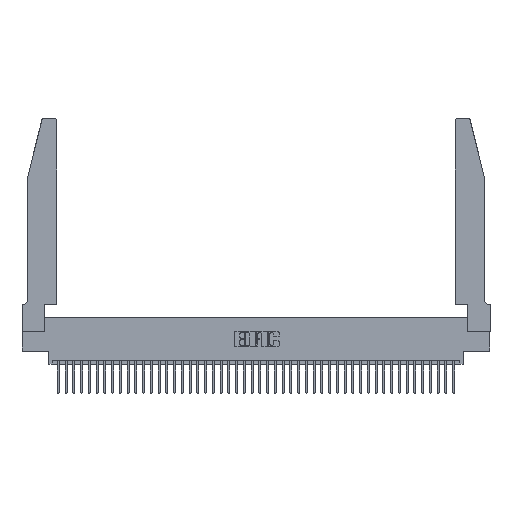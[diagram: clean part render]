
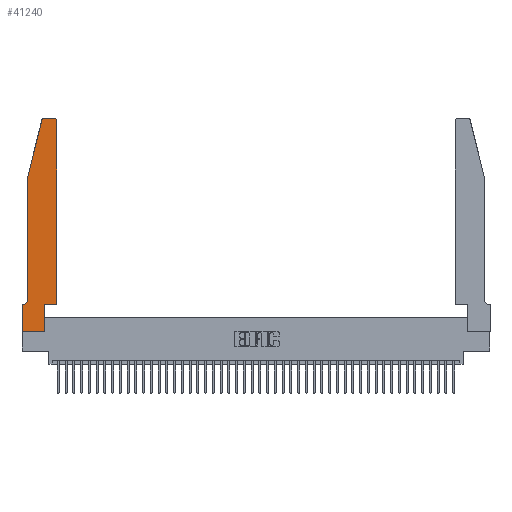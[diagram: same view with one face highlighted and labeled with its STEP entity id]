
A CAD part, top view. The second image highlights one B-rep face of the part: STEP entity #41240.
In plain terms, the highlighted planar face has unit normal (0, 0, 1).
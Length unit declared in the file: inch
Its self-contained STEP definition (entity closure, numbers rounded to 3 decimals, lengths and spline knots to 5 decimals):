
#177 = DIRECTION ( 'NONE',  ( 0., 1., 0. ) ) ;
#763 = DIRECTION ( 'NONE',  ( -0.239, -0.971, 0. ) ) ;
#1965 = CIRCLE ( 'NONE', #7921, 0.07 ) ;
#2280 = VERTEX_POINT ( 'NONE', #5767 ) ;
#2513 = ORIENTED_EDGE ( 'NONE', *, *, #29486, .T. ) ;
#2930 = DIRECTION ( 'NONE',  ( 1., 0., 0. ) ) ;
#3044 = FACE_OUTER_BOUND ( 'NONE', #36566, .T. ) ;
#3573 = AXIS2_PLACEMENT_3D ( 'NONE', #9579, #36799, #13159 ) ;
#3617 = VECTOR ( 'NONE', #177, 39.37008 ) ;
#3739 = EDGE_CURVE ( 'NONE', #2280, #36924, #19705, .T. ) ;
#4438 = CARTESIAN_POINT ( 'NONE',  ( 0.2605, 2.75, 0.37 ) ) ;
#4648 = ORIENTED_EDGE ( 'NONE', *, *, #14886, .T. ) ;
#5767 = CARTESIAN_POINT ( 'NONE',  ( 0.284, 2.75, 0.37 ) ) ;
#5982 = EDGE_CURVE ( 'NONE', #24374, #2280, #41078, .T. ) ;
#6125 = ORIENTED_EDGE ( 'NONE', *, *, #11329, .T. ) ;
#6128 = ORIENTED_EDGE ( 'NONE', *, *, #5982, .T. ) ;
#7256 = CARTESIAN_POINT ( 'NONE',  ( 0.4205, 2.72, 0.37 ) ) ;
#7770 = CARTESIAN_POINT ( 'NONE',  ( 0., 0., 0.37 ) ) ;
#7921 = AXIS2_PLACEMENT_3D ( 'NONE', #29848, #9232, #20041 ) ;
#8768 = ORIENTED_EDGE ( 'NONE', *, *, #29481, .T. ) ;
#9021 = CARTESIAN_POINT ( 'NONE',  ( 0.0055, 0.35, 0.37 ) ) ;
#9183 = VECTOR ( 'NONE', #14532, 39.37008 ) ;
#9232 = DIRECTION ( 'NONE',  ( 0., 0., -1. ) ) ;
#9338 = VECTOR ( 'NONE', #35047, 39.37008 ) ;
#9579 = CARTESIAN_POINT ( 'NONE',  ( 0., 0.35, 0.37 ) ) ;
#9632 = CARTESIAN_POINT ( 'NONE',  ( 0.284, 2.72, 0.37 ) ) ;
#9976 = VECTOR ( 'NONE', #16773, 39.37008 ) ;
#10547 = LINE ( 'NONE', #24568, #3617 ) ;
#10898 = CARTESIAN_POINT ( 'NONE',  ( 0.4505, 0.35, 0.37 ) ) ;
#11329 = EDGE_CURVE ( 'NONE', #16877, #13944, #31645, .T. ) ;
#12006 = DIRECTION ( 'NONE',  ( 1., 0., 0. ) ) ;
#12600 = ORIENTED_EDGE ( 'NONE', *, *, #39792, .T. ) ;
#13052 = CARTESIAN_POINT ( 'NONE',  ( 0.4505, 2.72, 0.37 ) ) ;
#13159 = DIRECTION ( 'NONE',  ( 1., 0., 0. ) ) ;
#13393 = EDGE_CURVE ( 'NONE', #20258, #36377, #28269, .T. ) ;
#13695 = EDGE_CURVE ( 'NONE', #18175, #24374, #19081, .T. ) ;
#13944 = VERTEX_POINT ( 'NONE', #23551 ) ;
#14532 = DIRECTION ( 'NONE',  ( 1., 0., 0. ) ) ;
#14886 = EDGE_CURVE ( 'NONE', #36924, #16877, #23790, .T. ) ;
#15280 = EDGE_CURVE ( 'NONE', #21926, #24134, #31861, .T. ) ;
#15755 = ORIENTED_EDGE ( 'NONE', *, *, #3739, .T. ) ;
#16176 = PLANE ( 'NONE',  #3573 ) ;
#16332 = CARTESIAN_POINT ( 'NONE',  ( 0.2865, 0.35, 0.37 ) ) ;
#16531 = DIRECTION ( 'NONE',  ( 0., 0., 1. ) ) ;
#16773 = DIRECTION ( 'NONE',  ( 0., -1., 0. ) ) ;
#16877 = VERTEX_POINT ( 'NONE', #39538 ) ;
#17230 = LINE ( 'NONE', #27946, #43605 ) ;
#17723 = DIRECTION ( 'NONE',  ( 0., -1., 0. ) ) ;
#18175 = VERTEX_POINT ( 'NONE', #13052 ) ;
#18686 = LINE ( 'NONE', #44092, #29438 ) ;
#19081 = CIRCLE ( 'NONE', #23054, 0.03 ) ;
#19705 = CIRCLE ( 'NONE', #37170, 0.03 ) ;
#20041 = DIRECTION ( 'NONE',  ( -1., 0., 0. ) ) ;
#20258 = VERTEX_POINT ( 'NONE', #42722 ) ;
#20551 = CARTESIAN_POINT ( 'NONE',  ( 0.0755, 2., 0.37 ) ) ;
#21791 = CARTESIAN_POINT ( 'NONE',  ( 0., 0., 0.37 ) ) ;
#21926 = VERTEX_POINT ( 'NONE', #16332 ) ;
#23054 = AXIS2_PLACEMENT_3D ( 'NONE', #7256, #34782, #35682 ) ;
#23511 = DIRECTION ( 'NONE',  ( 0., 1., 0. ) ) ;
#23551 = CARTESIAN_POINT ( 'NONE',  ( 0.0755, 0.42, 0.37 ) ) ;
#23790 = LINE ( 'NONE', #20551, #32983 ) ;
#23934 = ORIENTED_EDGE ( 'NONE', *, *, #31470, .T. ) ;
#24134 = VERTEX_POINT ( 'NONE', #10898 ) ;
#24374 = VERTEX_POINT ( 'NONE', #44344 ) ;
#24568 = CARTESIAN_POINT ( 'NONE',  ( 0.2865, 0.35, 0.37 ) ) ;
#24675 = CARTESIAN_POINT ( 'NONE',  ( 0.2865, 0., 0.37 ) ) ;
#27946 = CARTESIAN_POINT ( 'NONE',  ( 0.0755, 0.35, 0.37 ) ) ;
#28269 = LINE ( 'NONE', #21791, #9976 ) ;
#29017 = VERTEX_POINT ( 'NONE', #9021 ) ;
#29438 = VECTOR ( 'NONE', #23511, 39.37008 ) ;
#29481 = EDGE_CURVE ( 'NONE', #36377, #37327, #30169, .T. ) ;
#29486 = EDGE_CURVE ( 'NONE', #29017, #20258, #17230, .T. ) ;
#29848 = CARTESIAN_POINT ( 'NONE',  ( 0.0055, 0.42, 0.37 ) ) ;
#30169 = LINE ( 'NONE', #7770, #9183 ) ;
#30491 = ORIENTED_EDGE ( 'NONE', *, *, #15280, .T. ) ;
#31154 = ORIENTED_EDGE ( 'NONE', *, *, #13393, .T. ) ;
#31470 = EDGE_CURVE ( 'NONE', #24134, #18175, #18686, .T. ) ;
#31645 = LINE ( 'NONE', #35325, #40231 ) ;
#31861 = LINE ( 'NONE', #35913, #36681 ) ;
#32872 = CARTESIAN_POINT ( 'NONE',  ( 0.25487, 2.72718, 0.37 ) ) ;
#32983 = VECTOR ( 'NONE', #763, 39.37008 ) ;
#33274 = EDGE_CURVE ( 'NONE', #13944, #29017, #1965, .T. ) ;
#34782 = DIRECTION ( 'NONE',  ( 0., 0., 1. ) ) ;
#35047 = DIRECTION ( 'NONE',  ( -1., 0., 0. ) ) ;
#35325 = CARTESIAN_POINT ( 'NONE',  ( 0.0755, 2., 0.37 ) ) ;
#35682 = DIRECTION ( 'NONE',  ( 1., 0., 0. ) ) ;
#35913 = CARTESIAN_POINT ( 'NONE',  ( 0.4505, 0.35, 0.37 ) ) ;
#36377 = VERTEX_POINT ( 'NONE', #39497 ) ;
#36566 = EDGE_LOOP ( 'NONE', ( #6128, #15755, #4648, #6125, #42005, #2513, #31154, #8768, #12600, #30491, #23934, #40653 ) ) ;
#36681 = VECTOR ( 'NONE', #12006, 39.37008 ) ;
#36799 = DIRECTION ( 'NONE',  ( 0., 0., 1. ) ) ;
#36924 = VERTEX_POINT ( 'NONE', #32872 ) ;
#37170 = AXIS2_PLACEMENT_3D ( 'NONE', #9632, #16531, #2930 ) ;
#37327 = VERTEX_POINT ( 'NONE', #24675 ) ;
#39497 = CARTESIAN_POINT ( 'NONE',  ( 0., 0., 0.37 ) ) ;
#39538 = CARTESIAN_POINT ( 'NONE',  ( 0.0755, 2., 0.37 ) ) ;
#39792 = EDGE_CURVE ( 'NONE', #37327, #21926, #10547, .T. ) ;
#40231 = VECTOR ( 'NONE', #17723, 39.37008 ) ;
#40653 = ORIENTED_EDGE ( 'NONE', *, *, #13695, .T. ) ;
#41078 = LINE ( 'NONE', #4438, #9338 ) ;
#41240 = ADVANCED_FACE ( 'NONE', ( #3044 ), #16176, .T. ) ;
#41595 = DIRECTION ( 'NONE',  ( -1., 0., 0. ) ) ;
#42005 = ORIENTED_EDGE ( 'NONE', *, *, #33274, .T. ) ;
#42722 = CARTESIAN_POINT ( 'NONE',  ( 0., 0.35, 0.37 ) ) ;
#43605 = VECTOR ( 'NONE', #41595, 39.37008 ) ;
#44092 = CARTESIAN_POINT ( 'NONE',  ( 0.4505, 0.35, 0.37 ) ) ;
#44344 = CARTESIAN_POINT ( 'NONE',  ( 0.4205, 2.75, 0.37 ) ) ;
